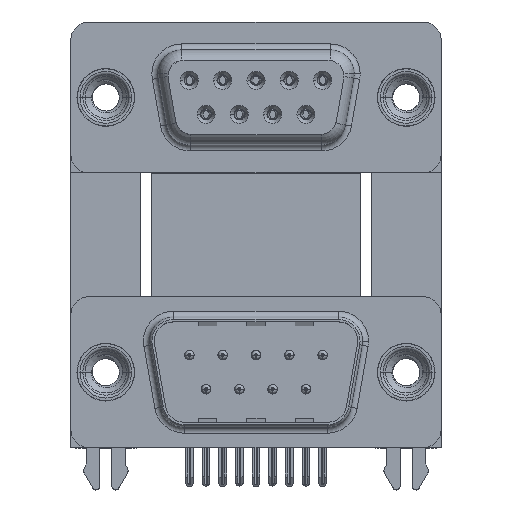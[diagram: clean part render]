
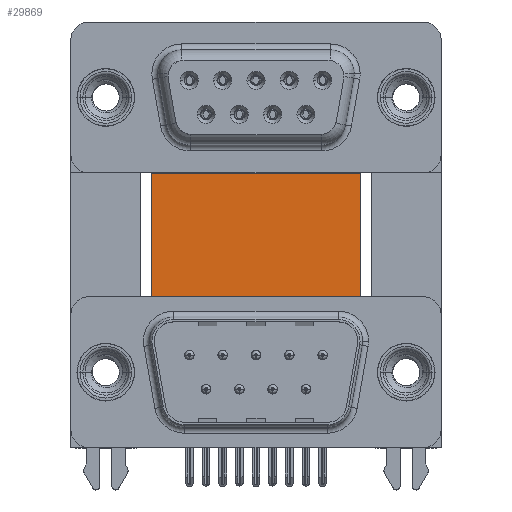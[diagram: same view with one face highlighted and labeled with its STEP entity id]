
A CAD part, top view. The second image highlights one B-rep face of the part: STEP entity #29869.
In plain terms, the highlighted planar face has unit normal (0, 0, 1).
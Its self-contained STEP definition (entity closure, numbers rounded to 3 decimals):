
#90 = VERTEX_POINT ( 'NONE', #1404 ) ;
#117 = DIRECTION ( 'NONE',  ( 1., 0., 0. ) ) ;
#330 = ORIENTED_EDGE ( 'NONE', *, *, #9428, .F. ) ;
#1324 = CARTESIAN_POINT ( 'NONE',  ( 2.9, -3.735, -12. ) ) ;
#1404 = CARTESIAN_POINT ( 'NONE',  ( 22.09, -3.735, -12. ) ) ;
#1411 = ORIENTED_EDGE ( 'NONE', *, *, #8365, .T. ) ;
#1639 = EDGE_CURVE ( 'NONE', #13876, #17109, #37213, .T. ) ;
#2526 = DIRECTION ( 'NONE',  ( -1., 0., 0. ) ) ;
#2541 = VECTOR ( 'NONE', #4736, 1000. ) ;
#3005 = VECTOR ( 'NONE', #15825, 1000. ) ;
#3454 = VECTOR ( 'NONE', #3737, 1000. ) ;
#3535 = LINE ( 'NONE', #31366, #3454 ) ;
#3737 = DIRECTION ( 'NONE',  ( -0.336, 0.942, 0. ) ) ;
#4736 = DIRECTION ( 'NONE',  ( 1., 0., 0. ) ) ;
#6563 = EDGE_CURVE ( 'NONE', #20366, #39149, #30915, .T. ) ;
#7237 = VERTEX_POINT ( 'NONE', #11988 ) ;
#8365 = EDGE_CURVE ( 'NONE', #7237, #20366, #26122, .T. ) ;
#9354 = CARTESIAN_POINT ( 'NONE',  ( 2.9, -3.735, -12. ) ) ;
#9428 = EDGE_CURVE ( 'NONE', #13876, #38342, #11057, .T. ) ;
#9799 = LINE ( 'NONE', #22080, #12914 ) ;
#10333 = CARTESIAN_POINT ( 'NONE',  ( 22.09, -4.635, -12. ) ) ;
#10607 = EDGE_LOOP ( 'NONE', ( #12499, #12702, #20229, #12888, #16303, #330, #36599, #35505, #1411, #15794 ) ) ;
#11057 = LINE ( 'NONE', #20515, #34160 ) ;
#11625 = DIRECTION ( 'NONE',  ( 0., 0., -1. ) ) ;
#11988 = CARTESIAN_POINT ( 'NONE',  ( 2.4, -4.635, -12. ) ) ;
#12499 = ORIENTED_EDGE ( 'NONE', *, *, #35845, .T. ) ;
#12532 = LINE ( 'NONE', #24804, #28208 ) ;
#12672 = DIRECTION ( 'NONE',  ( -0.336, -0.942, 0. ) ) ;
#12702 = ORIENTED_EDGE ( 'NONE', *, *, #21127, .T. ) ;
#12888 = ORIENTED_EDGE ( 'NONE', *, *, #22088, .T. ) ;
#12914 = VECTOR ( 'NONE', #117, 1000. ) ;
#13876 = VERTEX_POINT ( 'NONE', #29822 ) ;
#14927 = VERTEX_POINT ( 'NONE', #26681 ) ;
#15794 = ORIENTED_EDGE ( 'NONE', *, *, #6563, .T. ) ;
#15825 = DIRECTION ( 'NONE',  ( 0., -1., 0. ) ) ;
#16303 = ORIENTED_EDGE ( 'NONE', *, *, #24314, .F. ) ;
#17082 = PLANE ( 'NONE',  #30059 ) ;
#17109 = VERTEX_POINT ( 'NONE', #38877 ) ;
#19050 = LINE ( 'NONE', #31336, #26749 ) ;
#19925 = CARTESIAN_POINT ( 'NONE',  ( 22.59, -4.635, -12. ) ) ;
#20229 = ORIENTED_EDGE ( 'NONE', *, *, #33194, .T. ) ;
#20366 = VERTEX_POINT ( 'NONE', #24599 ) ;
#20515 = CARTESIAN_POINT ( 'NONE',  ( 3.79, 16.585, -12. ) ) ;
#21127 = EDGE_CURVE ( 'NONE', #90, #31905, #36179, .T. ) ;
#21439 = VECTOR ( 'NONE', #21631, 1000. ) ;
#21631 = DIRECTION ( 'NONE',  ( 0., 1., 0. ) ) ;
#21879 = CARTESIAN_POINT ( 'NONE',  ( 3.79, 16.585, -12. ) ) ;
#22080 = CARTESIAN_POINT ( 'NONE',  ( 3.79, -3.735, -12. ) ) ;
#22088 = EDGE_CURVE ( 'NONE', #38654, #14927, #3535, .T. ) ;
#22117 = LINE ( 'NONE', #27972, #39052 ) ;
#23339 = DIRECTION ( 'NONE',  ( 1., 0., 0. ) ) ;
#24314 = EDGE_CURVE ( 'NONE', #38342, #14927, #19050, .T. ) ;
#24599 = CARTESIAN_POINT ( 'NONE',  ( 2.9, -4.635, -12. ) ) ;
#24804 = CARTESIAN_POINT ( 'NONE',  ( 22.09, -4.635, -12. ) ) ;
#26122 = LINE ( 'NONE', #38420, #2541 ) ;
#26317 = DIRECTION ( 'NONE',  ( 0., -1., 0. ) ) ;
#26681 = CARTESIAN_POINT ( 'NONE',  ( 21.2, -0.735, -12. ) ) ;
#26749 = VECTOR ( 'NONE', #37593, 1000. ) ;
#26942 = FACE_OUTER_BOUND ( 'NONE', #10607, .T. ) ;
#27972 = CARTESIAN_POINT ( 'NONE',  ( 2.4, -4.635, -12. ) ) ;
#28208 = VECTOR ( 'NONE', #34082, 1000. ) ;
#29574 = EDGE_CURVE ( 'NONE', #17109, #7237, #22117, .T. ) ;
#29822 = CARTESIAN_POINT ( 'NONE',  ( 3.79, 16.585, -12. ) ) ;
#29869 = ADVANCED_FACE ( 'NONE', ( #26942 ), #17082, .F. ) ;
#30059 = AXIS2_PLACEMENT_3D ( 'NONE', #39221, #11625, #2526 ) ;
#30834 = CARTESIAN_POINT ( 'NONE',  ( 21.2, 16.585, -12. ) ) ;
#30915 = LINE ( 'NONE', #9354, #21439 ) ;
#31336 = CARTESIAN_POINT ( 'NONE',  ( 21.2, 16.585, -12. ) ) ;
#31366 = CARTESIAN_POINT ( 'NONE',  ( 22.59, -4.635, -12. ) ) ;
#31905 = VERTEX_POINT ( 'NONE', #10333 ) ;
#32359 = CARTESIAN_POINT ( 'NONE',  ( 22.09, -3.735, -12. ) ) ;
#32655 = VECTOR ( 'NONE', #26317, 1000. ) ;
#33194 = EDGE_CURVE ( 'NONE', #31905, #38654, #12532, .T. ) ;
#34082 = DIRECTION ( 'NONE',  ( 1., 0., 0. ) ) ;
#34160 = VECTOR ( 'NONE', #23339, 1000. ) ;
#35505 = ORIENTED_EDGE ( 'NONE', *, *, #29574, .T. ) ;
#35845 = EDGE_CURVE ( 'NONE', #39149, #90, #9799, .T. ) ;
#36179 = LINE ( 'NONE', #32359, #32655 ) ;
#36599 = ORIENTED_EDGE ( 'NONE', *, *, #1639, .T. ) ;
#37213 = LINE ( 'NONE', #21879, #3005 ) ;
#37593 = DIRECTION ( 'NONE',  ( 0., -1., 0. ) ) ;
#38342 = VERTEX_POINT ( 'NONE', #30834 ) ;
#38420 = CARTESIAN_POINT ( 'NONE',  ( 2.9, -4.635, -12. ) ) ;
#38654 = VERTEX_POINT ( 'NONE', #19925 ) ;
#38877 = CARTESIAN_POINT ( 'NONE',  ( 3.79, -0.735, -12. ) ) ;
#39052 = VECTOR ( 'NONE', #12672, 1000. ) ;
#39149 = VERTEX_POINT ( 'NONE', #1324 ) ;
#39221 = CARTESIAN_POINT ( 'NONE',  ( 3.79, 16.585, -12. ) ) ;
